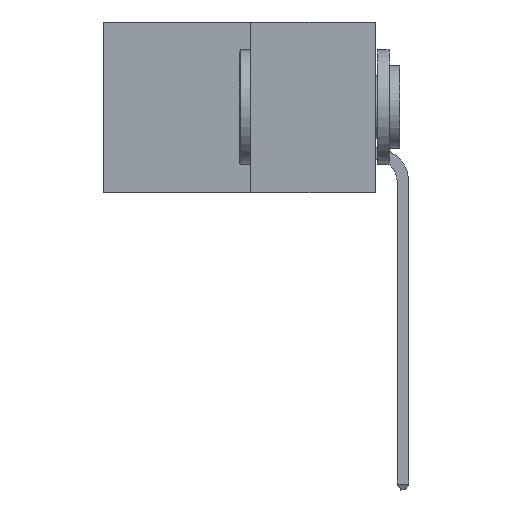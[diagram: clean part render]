
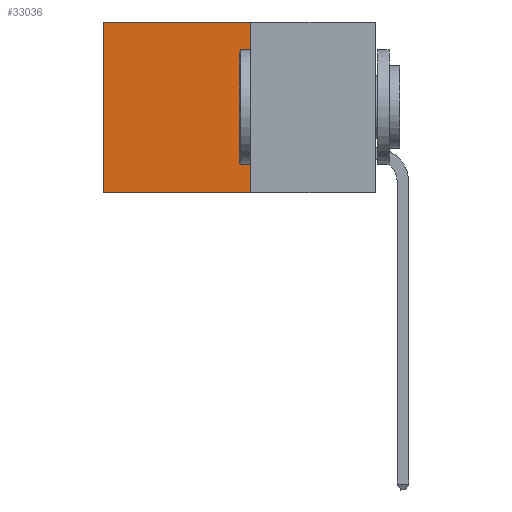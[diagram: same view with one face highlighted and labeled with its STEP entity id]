
A CAD part, left-side view. The second image highlights one B-rep face of the part: STEP entity #33036.
In plain terms, the highlighted planar face has unit normal (-1, 0, 0).
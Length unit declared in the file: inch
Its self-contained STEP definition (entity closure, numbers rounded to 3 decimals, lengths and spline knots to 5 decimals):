
#7 = VERTEX_POINT ( 'NONE', #13516 ) ;
#31 = CARTESIAN_POINT ( 'NONE',  ( 0.277, 0.27, -0.37 ) ) ;
#228 = CARTESIAN_POINT ( 'NONE',  ( 0.277, 0.59, 0. ) ) ;
#875 = ORIENTED_EDGE ( 'NONE', *, *, #3265, .F. ) ;
#925 = CARTESIAN_POINT ( 'NONE',  ( 0.277, 0.59, -0.37 ) ) ;
#1756 = EDGE_CURVE ( 'NONE', #24872, #21250, #2099, .T. ) ;
#1995 = EDGE_LOOP ( 'NONE', ( #15237, #31388, #875, #27968 ) ) ;
#2099 = LINE ( 'NONE', #16870, #3759 ) ;
#2992 = LINE ( 'NONE', #29991, #16359 ) ;
#3265 = EDGE_CURVE ( 'NONE', #24872, #4689, #16234, .T. ) ;
#3474 = AXIS2_PLACEMENT_3D ( 'NONE', #31, #26553, #10743 ) ;
#3759 = VECTOR ( 'NONE', #21909, 39.37008 ) ;
#4689 = VERTEX_POINT ( 'NONE', #31593 ) ;
#8377 = VECTOR ( 'NONE', #19420, 39.37008 ) ;
#10317 = CARTESIAN_POINT ( 'NONE',  ( 0.277, 0.27, 0. ) ) ;
#10743 = DIRECTION ( 'NONE',  ( 0., 0., -1. ) ) ;
#13516 = CARTESIAN_POINT ( 'NONE',  ( 0.277, 0.59, -0.37 ) ) ;
#15237 = ORIENTED_EDGE ( 'NONE', *, *, #25874, .T. ) ;
#15982 = PLANE ( 'NONE',  #3474 ) ;
#16234 = LINE ( 'NONE', #17764, #30111 ) ;
#16359 = VECTOR ( 'NONE', #17022, 39.37008 ) ;
#16870 = CARTESIAN_POINT ( 'NONE',  ( 0.277, 0.27, 0. ) ) ;
#17022 = DIRECTION ( 'NONE',  ( 0., 1., 0. ) ) ;
#17764 = CARTESIAN_POINT ( 'NONE',  ( 0.277, 0.27, -0.37 ) ) ;
#17811 = DIRECTION ( 'NONE',  ( 0., 0., -1. ) ) ;
#19420 = DIRECTION ( 'NONE',  ( 0., 0., -1. ) ) ;
#19970 = EDGE_CURVE ( 'NONE', #4689, #7, #2992, .T. ) ;
#20539 = FACE_OUTER_BOUND ( 'NONE', #1995, .T. ) ;
#21250 = VERTEX_POINT ( 'NONE', #228 ) ;
#21909 = DIRECTION ( 'NONE',  ( 0., 1., 0. ) ) ;
#24872 = VERTEX_POINT ( 'NONE', #10317 ) ;
#25874 = EDGE_CURVE ( 'NONE', #21250, #7, #26653, .T. ) ;
#26553 = DIRECTION ( 'NONE',  ( 1., 0., 0. ) ) ;
#26653 = LINE ( 'NONE', #925, #8377 ) ;
#27968 = ORIENTED_EDGE ( 'NONE', *, *, #1756, .T. ) ;
#29991 = CARTESIAN_POINT ( 'NONE',  ( 0.277, 0.27, -0.37 ) ) ;
#30111 = VECTOR ( 'NONE', #17811, 39.37008 ) ;
#31388 = ORIENTED_EDGE ( 'NONE', *, *, #19970, .F. ) ;
#31593 = CARTESIAN_POINT ( 'NONE',  ( 0.277, 0.27, -0.37 ) ) ;
#33036 = ADVANCED_FACE ( 'NONE', ( #20539 ), #15982, .F. ) ;
